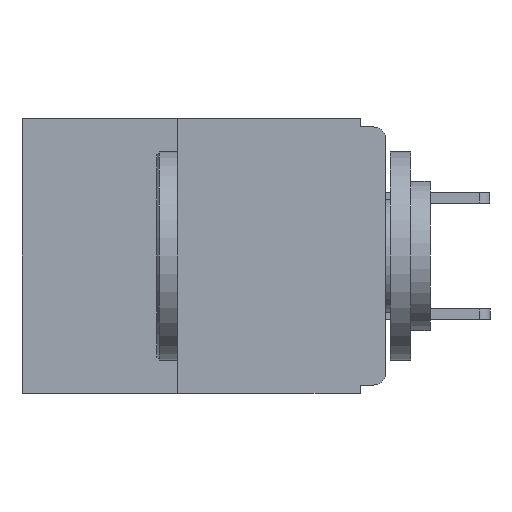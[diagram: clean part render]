
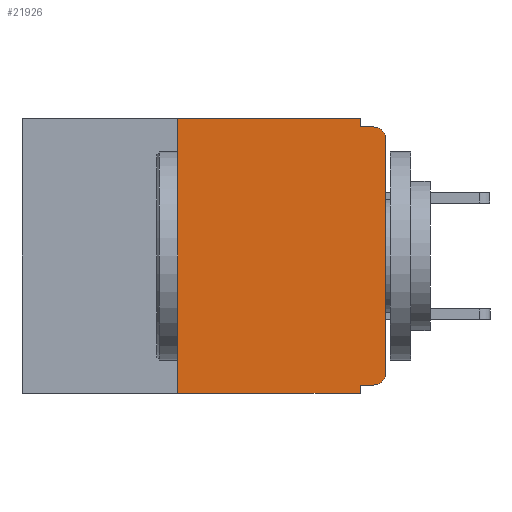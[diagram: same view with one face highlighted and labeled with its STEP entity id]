
A CAD part, left-side view. The second image highlights one B-rep face of the part: STEP entity #21926.
In plain terms, the highlighted planar face has unit normal (-1, 0, 0).
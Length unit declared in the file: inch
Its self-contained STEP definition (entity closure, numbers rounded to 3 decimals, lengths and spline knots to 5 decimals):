
#259 = CIRCLE ( 'NONE', #4627, 0.015 ) ;
#854 = CARTESIAN_POINT ( 'NONE',  ( 0., 0., -0.32 ) ) ;
#879 = VERTEX_POINT ( 'NONE', #20305 ) ;
#1409 = VERTEX_POINT ( 'NONE', #12938 ) ;
#2278 = LINE ( 'NONE', #10235, #13072 ) ;
#2483 = ORIENTED_EDGE ( 'NONE', *, *, #13308, .T. ) ;
#2567 = ORIENTED_EDGE ( 'NONE', *, *, #3994, .F. ) ;
#3119 = ORIENTED_EDGE ( 'NONE', *, *, #23865, .T. ) ;
#3181 = DIRECTION ( 'NONE',  ( 0., 0., 1. ) ) ;
#3372 = CARTESIAN_POINT ( 'NONE',  ( 0., 0.25, -0.33 ) ) ;
#3994 = EDGE_CURVE ( 'NONE', #14014, #4743, #21433, .T. ) ;
#4187 = EDGE_CURVE ( 'NONE', #879, #17608, #27627, .T. ) ;
#4627 = AXIS2_PLACEMENT_3D ( 'NONE', #20033, #6319, #22249 ) ;
#4743 = VERTEX_POINT ( 'NONE', #5302 ) ;
#4840 = CARTESIAN_POINT ( 'NONE',  ( 0., 0.015, -0.305 ) ) ;
#5266 = ORIENTED_EDGE ( 'NONE', *, *, #20948, .F. ) ;
#5302 = CARTESIAN_POINT ( 'NONE',  ( 0., 0.031, -0.01 ) ) ;
#6319 = DIRECTION ( 'NONE',  ( -1., 0., 0. ) ) ;
#6524 = FACE_OUTER_BOUND ( 'NONE', #12771, .T. ) ;
#6619 = PLANE ( 'NONE',  #11980 ) ;
#7127 = CARTESIAN_POINT ( 'NONE',  ( 0., 0.437, -0.33 ) ) ;
#7171 = DIRECTION ( 'NONE',  ( 0., 0., -1. ) ) ;
#7371 = VECTOR ( 'NONE', #23067, 39.37008 ) ;
#7580 = VERTEX_POINT ( 'NONE', #20073 ) ;
#9029 = LINE ( 'NONE', #3372, #21171 ) ;
#9062 = CARTESIAN_POINT ( 'NONE',  ( 0., 0.031, -0.33 ) ) ;
#9483 = LINE ( 'NONE', #28535, #20904 ) ;
#10046 = DIRECTION ( 'NONE',  ( 0., 1., 0. ) ) ;
#10235 = CARTESIAN_POINT ( 'NONE',  ( 0., 0.437, 0. ) ) ;
#10460 = EDGE_CURVE ( 'NONE', #17608, #1409, #259, .T. ) ;
#11156 = CARTESIAN_POINT ( 'NONE',  ( 0., 0.031, -0.32 ) ) ;
#11249 = DIRECTION ( 'NONE',  ( 0., 0., -1. ) ) ;
#11980 = AXIS2_PLACEMENT_3D ( 'NONE', #22562, #24800, #11249 ) ;
#12029 = ORIENTED_EDGE ( 'NONE', *, *, #4187, .T. ) ;
#12744 = CARTESIAN_POINT ( 'NONE',  ( 0., 0.031, -0.33 ) ) ;
#12771 = EDGE_LOOP ( 'NONE', ( #12029, #16000, #5266, #2567, #13077, #27398, #3119, #22783, #20707, #2483 ) ) ;
#12938 = CARTESIAN_POINT ( 'NONE',  ( 0., 0.015, -0.01 ) ) ;
#12956 = DIRECTION ( 'NONE',  ( 0., -1., 0. ) ) ;
#13072 = VECTOR ( 'NONE', #23917, 39.37008 ) ;
#13077 = ORIENTED_EDGE ( 'NONE', *, *, #14176, .F. ) ;
#13308 = EDGE_CURVE ( 'NONE', #7580, #879, #18548, .T. ) ;
#14014 = VERTEX_POINT ( 'NONE', #25482 ) ;
#14176 = EDGE_CURVE ( 'NONE', #26763, #14014, #2278, .T. ) ;
#14621 = CARTESIAN_POINT ( 'NONE',  ( 0., 0.25, 0. ) ) ;
#15727 = VECTOR ( 'NONE', #3181, 39.37008 ) ;
#16000 = ORIENTED_EDGE ( 'NONE', *, *, #10460, .T. ) ;
#16225 = CARTESIAN_POINT ( 'NONE',  ( 0., 0.25, -0.33 ) ) ;
#16331 = EDGE_CURVE ( 'NONE', #22688, #26763, #9029, .T. ) ;
#16552 = VECTOR ( 'NONE', #26273, 39.37008 ) ;
#17608 = VERTEX_POINT ( 'NONE', #28142 ) ;
#18548 = CIRCLE ( 'NONE', #28702, 0.015 ) ;
#18593 = DIRECTION ( 'NONE',  ( 0., 0., -1. ) ) ;
#19283 = CARTESIAN_POINT ( 'NONE',  ( 0., 0., 0. ) ) ;
#20033 = CARTESIAN_POINT ( 'NONE',  ( 0., 0.015, -0.025 ) ) ;
#20037 = VECTOR ( 'NONE', #18593, 39.37008 ) ;
#20073 = CARTESIAN_POINT ( 'NONE',  ( 0., 0.015, -0.32 ) ) ;
#20305 = CARTESIAN_POINT ( 'NONE',  ( 0., 0., -0.305 ) ) ;
#20707 = ORIENTED_EDGE ( 'NONE', *, *, #22240, .F. ) ;
#20861 = DIRECTION ( 'NONE',  ( -1., 0., 0. ) ) ;
#20904 = VECTOR ( 'NONE', #12956, 39.37008 ) ;
#20948 = EDGE_CURVE ( 'NONE', #4743, #1409, #9483, .T. ) ;
#21171 = VECTOR ( 'NONE', #23822, 39.37008 ) ;
#21433 = LINE ( 'NONE', #25308, #20037 ) ;
#21926 = ADVANCED_FACE ( 'NONE', ( #6524 ), #6619, .F. ) ;
#22197 = LINE ( 'NONE', #854, #27378 ) ;
#22240 = EDGE_CURVE ( 'NONE', #7580, #23735, #22197, .T. ) ;
#22249 = DIRECTION ( 'NONE',  ( 0., 0., -1. ) ) ;
#22543 = LINE ( 'NONE', #12744, #16552 ) ;
#22562 = CARTESIAN_POINT ( 'NONE',  ( 0., 0.437, 0. ) ) ;
#22688 = VERTEX_POINT ( 'NONE', #16225 ) ;
#22783 = ORIENTED_EDGE ( 'NONE', *, *, #26815, .F. ) ;
#23067 = DIRECTION ( 'NONE',  ( 0., -1., 0. ) ) ;
#23735 = VERTEX_POINT ( 'NONE', #11156 ) ;
#23822 = DIRECTION ( 'NONE',  ( 0., 0., 1. ) ) ;
#23865 = EDGE_CURVE ( 'NONE', #22688, #27031, #25468, .T. ) ;
#23917 = DIRECTION ( 'NONE',  ( 0., -1., 0. ) ) ;
#24800 = DIRECTION ( 'NONE',  ( 1., 0., 0. ) ) ;
#25308 = CARTESIAN_POINT ( 'NONE',  ( 0., 0.031, 0. ) ) ;
#25468 = LINE ( 'NONE', #7127, #7371 ) ;
#25482 = CARTESIAN_POINT ( 'NONE',  ( 0., 0.031, 0. ) ) ;
#26273 = DIRECTION ( 'NONE',  ( 0., 0., -1. ) ) ;
#26763 = VERTEX_POINT ( 'NONE', #14621 ) ;
#26815 = EDGE_CURVE ( 'NONE', #23735, #27031, #22543, .T. ) ;
#27031 = VERTEX_POINT ( 'NONE', #9062 ) ;
#27378 = VECTOR ( 'NONE', #10046, 39.37008 ) ;
#27398 = ORIENTED_EDGE ( 'NONE', *, *, #16331, .F. ) ;
#27627 = LINE ( 'NONE', #19283, #15727 ) ;
#28142 = CARTESIAN_POINT ( 'NONE',  ( 0., 0., -0.025 ) ) ;
#28535 = CARTESIAN_POINT ( 'NONE',  ( 0., 0., -0.01 ) ) ;
#28702 = AXIS2_PLACEMENT_3D ( 'NONE', #4840, #20861, #7171 ) ;
